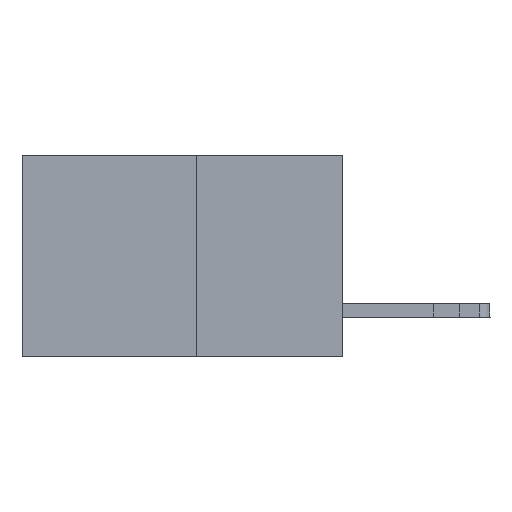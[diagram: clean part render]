
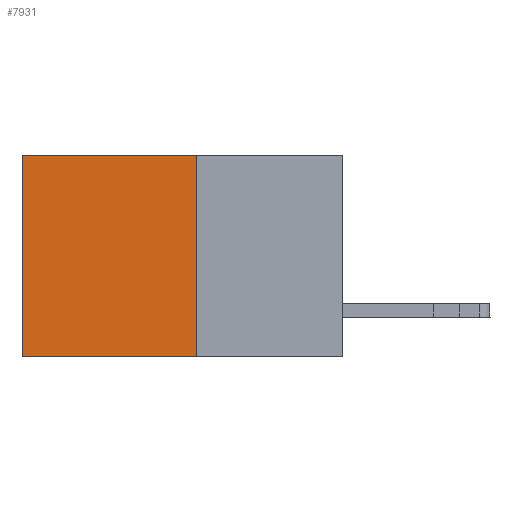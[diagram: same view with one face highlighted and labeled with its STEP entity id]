
A CAD part, left-side view. The second image highlights one B-rep face of the part: STEP entity #7931.
In plain terms, the highlighted planar face has unit normal (-1, 0, 0).
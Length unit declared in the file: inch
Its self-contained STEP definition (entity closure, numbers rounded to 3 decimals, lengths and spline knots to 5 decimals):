
#683 = EDGE_CURVE ( 'NONE', #16809, #13427, #18430, .T. ) ;
#1906 = EDGE_CURVE ( 'NONE', #16809, #16668, #10625, .T. ) ;
#2420 = DIRECTION ( 'NONE',  ( 0., 1., 0. ) ) ;
#2768 = ORIENTED_EDGE ( 'NONE', *, *, #7554, .F. ) ;
#4303 = VECTOR ( 'NONE', #2420, 39.37008 ) ;
#7135 = DIRECTION ( 'NONE',  ( 0., 1., 0. ) ) ;
#7222 = CARTESIAN_POINT ( 'NONE',  ( 0.277, 0.27, -0.37 ) ) ;
#7554 = EDGE_CURVE ( 'NONE', #16668, #11093, #8673, .T. ) ;
#7931 = ADVANCED_FACE ( 'NONE', ( #10711 ), #16883, .F. ) ;
#8093 = CARTESIAN_POINT ( 'NONE',  ( 0.277, 0.59, 0. ) ) ;
#8590 = ORIENTED_EDGE ( 'NONE', *, *, #1906, .F. ) ;
#8673 = LINE ( 'NONE', #15893, #16405 ) ;
#9166 = LINE ( 'NONE', #13887, #13323 ) ;
#9182 = DIRECTION ( 'NONE',  ( 0., 0., -1. ) ) ;
#9763 = ORIENTED_EDGE ( 'NONE', *, *, #683, .T. ) ;
#10625 = LINE ( 'NONE', #14968, #15704 ) ;
#10711 = FACE_OUTER_BOUND ( 'NONE', #10989, .T. ) ;
#10926 = CARTESIAN_POINT ( 'NONE',  ( 0.277, 0.27, 0. ) ) ;
#10989 = EDGE_LOOP ( 'NONE', ( #16448, #2768, #8590, #9763 ) ) ;
#11093 = VERTEX_POINT ( 'NONE', #18579 ) ;
#13143 = DIRECTION ( 'NONE',  ( 0., 0., -1. ) ) ;
#13323 = VECTOR ( 'NONE', #16481, 39.37008 ) ;
#13427 = VERTEX_POINT ( 'NONE', #8093 ) ;
#13670 = EDGE_CURVE ( 'NONE', #13427, #11093, #9166, .T. ) ;
#13887 = CARTESIAN_POINT ( 'NONE',  ( 0.277, 0.59, -0.37 ) ) ;
#14968 = CARTESIAN_POINT ( 'NONE',  ( 0.277, 0.27, -0.37 ) ) ;
#15196 = CARTESIAN_POINT ( 'NONE',  ( 0.277, 0.27, 0. ) ) ;
#15447 = DIRECTION ( 'NONE',  ( 1., 0., 0. ) ) ;
#15704 = VECTOR ( 'NONE', #13143, 39.37008 ) ;
#15893 = CARTESIAN_POINT ( 'NONE',  ( 0.277, 0.27, -0.37 ) ) ;
#16116 = AXIS2_PLACEMENT_3D ( 'NONE', #16591, #15447, #9182 ) ;
#16405 = VECTOR ( 'NONE', #7135, 39.37008 ) ;
#16448 = ORIENTED_EDGE ( 'NONE', *, *, #13670, .T. ) ;
#16481 = DIRECTION ( 'NONE',  ( 0., 0., -1. ) ) ;
#16591 = CARTESIAN_POINT ( 'NONE',  ( 0.277, 0.27, -0.37 ) ) ;
#16668 = VERTEX_POINT ( 'NONE', #7222 ) ;
#16809 = VERTEX_POINT ( 'NONE', #15196 ) ;
#16883 = PLANE ( 'NONE',  #16116 ) ;
#18430 = LINE ( 'NONE', #10926, #4303 ) ;
#18579 = CARTESIAN_POINT ( 'NONE',  ( 0.277, 0.59, -0.37 ) ) ;
